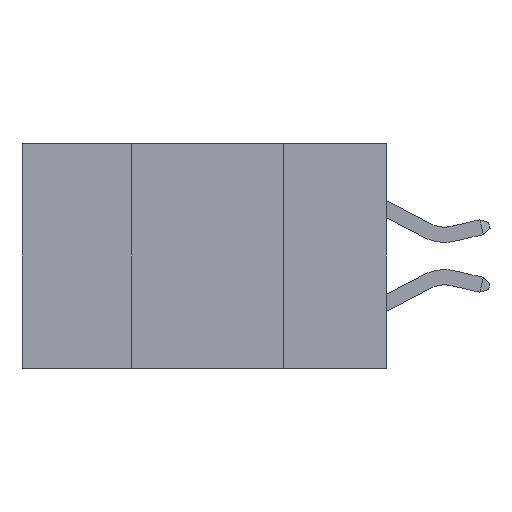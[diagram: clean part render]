
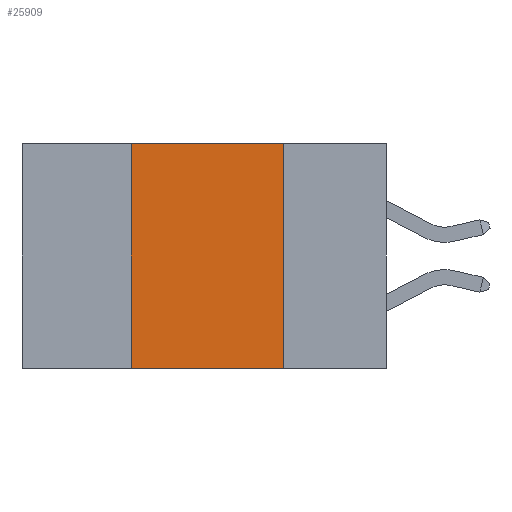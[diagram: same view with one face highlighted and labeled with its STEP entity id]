
A CAD part, left-side view. The second image highlights one B-rep face of the part: STEP entity #25909.
In plain terms, the highlighted planar face has unit normal (-1, 0, 0).
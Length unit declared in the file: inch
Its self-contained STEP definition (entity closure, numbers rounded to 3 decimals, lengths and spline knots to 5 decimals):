
#798 = VECTOR ( 'NONE', #5247, 39.37008 ) ;
#1121 = CARTESIAN_POINT ( 'NONE',  ( 0., 0.17, -0.37 ) ) ;
#2249 = LINE ( 'NONE', #16904, #4692 ) ;
#4018 = DIRECTION ( 'NONE',  ( 0., -1., 0. ) ) ;
#4394 = DIRECTION ( 'NONE',  ( 0., 0., -1. ) ) ;
#4490 = VERTEX_POINT ( 'NONE', #14469 ) ;
#4531 = PLANE ( 'NONE',  #21367 ) ;
#4562 = LINE ( 'NONE', #21803, #798 ) ;
#4692 = VECTOR ( 'NONE', #25256, 39.37008 ) ;
#5247 = DIRECTION ( 'NONE',  ( 0., 0., 1. ) ) ;
#5871 = CARTESIAN_POINT ( 'NONE',  ( 0., 0.6, -0.37 ) ) ;
#6052 = VECTOR ( 'NONE', #4018, 39.37008 ) ;
#6444 = CARTESIAN_POINT ( 'NONE',  ( 0., 0.42, -0.37 ) ) ;
#6694 = VERTEX_POINT ( 'NONE', #6444 ) ;
#7699 = EDGE_CURVE ( 'NONE', #6694, #26920, #24617, .T. ) ;
#9116 = EDGE_LOOP ( 'NONE', ( #20293, #17919, #16283, #16634 ) ) ;
#10641 = DIRECTION ( 'NONE',  ( 0., -1., 0. ) ) ;
#11530 = EDGE_CURVE ( 'NONE', #4490, #26920, #2249, .T. ) ;
#11807 = EDGE_CURVE ( 'NONE', #21656, #4490, #16201, .T. ) ;
#13969 = CARTESIAN_POINT ( 'NONE',  ( 0., 0.42, 0. ) ) ;
#14469 = CARTESIAN_POINT ( 'NONE',  ( 0., 0.17, 0. ) ) ;
#16201 = LINE ( 'NONE', #18395, #6052 ) ;
#16283 = ORIENTED_EDGE ( 'NONE', *, *, #25426, .F. ) ;
#16634 = ORIENTED_EDGE ( 'NONE', *, *, #7699, .T. ) ;
#16844 = DIRECTION ( 'NONE',  ( 1., 0., 0. ) ) ;
#16904 = CARTESIAN_POINT ( 'NONE',  ( 0., 0.17, -0.37 ) ) ;
#17919 = ORIENTED_EDGE ( 'NONE', *, *, #11807, .F. ) ;
#18395 = CARTESIAN_POINT ( 'NONE',  ( 0., 0.6, 0. ) ) ;
#18912 = CARTESIAN_POINT ( 'NONE',  ( 0., 0.6, 0. ) ) ;
#20293 = ORIENTED_EDGE ( 'NONE', *, *, #11530, .F. ) ;
#20969 = FACE_OUTER_BOUND ( 'NONE', #9116, .T. ) ;
#21367 = AXIS2_PLACEMENT_3D ( 'NONE', #18912, #16844, #4394 ) ;
#21656 = VERTEX_POINT ( 'NONE', #13969 ) ;
#21803 = CARTESIAN_POINT ( 'NONE',  ( 0., 0.42, -0.37 ) ) ;
#23982 = VECTOR ( 'NONE', #10641, 39.37008 ) ;
#24617 = LINE ( 'NONE', #5871, #23982 ) ;
#25256 = DIRECTION ( 'NONE',  ( 0., 0., -1. ) ) ;
#25426 = EDGE_CURVE ( 'NONE', #6694, #21656, #4562, .T. ) ;
#25909 = ADVANCED_FACE ( 'NONE', ( #20969 ), #4531, .F. ) ;
#26920 = VERTEX_POINT ( 'NONE', #1121 ) ;
